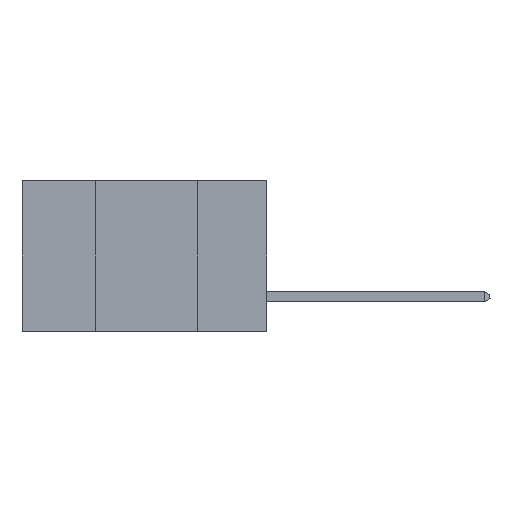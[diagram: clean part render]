
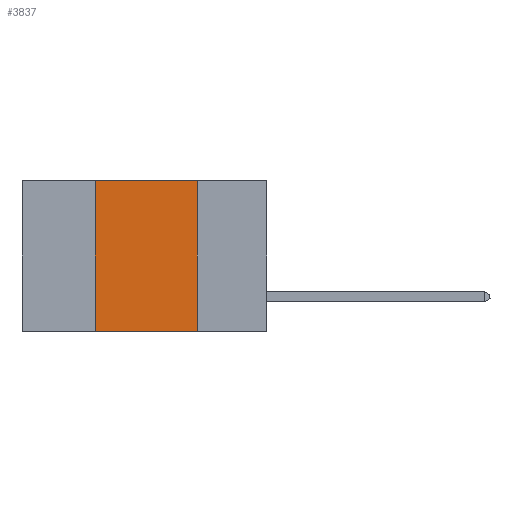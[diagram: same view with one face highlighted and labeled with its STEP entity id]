
A CAD part, left-side view. The second image highlights one B-rep face of the part: STEP entity #3837.
In plain terms, the highlighted planar face has unit normal (-1, 0, 0).
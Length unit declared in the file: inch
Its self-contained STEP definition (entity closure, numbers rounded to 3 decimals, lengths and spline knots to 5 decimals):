
#324 = CARTESIAN_POINT ( 'NONE',  ( 0., 0.42, 0. ) ) ;
#327 = CARTESIAN_POINT ( 'NONE',  ( 0., 0.42, -0.37 ) ) ;
#1622 = VECTOR ( 'NONE', #12497, 39.37008 ) ;
#2121 = CARTESIAN_POINT ( 'NONE',  ( 0., 0.17, 0. ) ) ;
#2590 = PLANE ( 'NONE',  #17501 ) ;
#3111 = ORIENTED_EDGE ( 'NONE', *, *, #18318, .F. ) ;
#3259 = CARTESIAN_POINT ( 'NONE',  ( 0., 0.42, 0. ) ) ;
#3837 = ADVANCED_FACE ( 'NONE', ( #7050 ), #2590, .F. ) ;
#4318 = VERTEX_POINT ( 'NONE', #2121 ) ;
#4724 = DIRECTION ( 'NONE',  ( 0., -1., 0. ) ) ;
#5685 = LINE ( 'NONE', #15489, #20625 ) ;
#5965 = LINE ( 'NONE', #324, #1622 ) ;
#6054 = DIRECTION ( 'NONE',  ( 0., 0., -1. ) ) ;
#6396 = LINE ( 'NONE', #6500, #17541 ) ;
#6500 = CARTESIAN_POINT ( 'NONE',  ( 0., 0.17, 0. ) ) ;
#7050 = FACE_OUTER_BOUND ( 'NONE', #10687, .T. ) ;
#7141 = VERTEX_POINT ( 'NONE', #3259 ) ;
#8416 = EDGE_CURVE ( 'NONE', #4318, #9882, #6396, .T. ) ;
#9678 = CARTESIAN_POINT ( 'NONE',  ( 0., 0.6, 0. ) ) ;
#9882 = VERTEX_POINT ( 'NONE', #21635 ) ;
#10262 = DIRECTION ( 'NONE',  ( 0., 0., -1. ) ) ;
#10321 = ORIENTED_EDGE ( 'NONE', *, *, #13271, .F. ) ;
#10687 = EDGE_LOOP ( 'NONE', ( #15034, #10321, #3111, #14745 ) ) ;
#12497 = DIRECTION ( 'NONE',  ( 0., 0., 1. ) ) ;
#13271 = EDGE_CURVE ( 'NONE', #7141, #4318, #19123, .T. ) ;
#14745 = ORIENTED_EDGE ( 'NONE', *, *, #18659, .T. ) ;
#15034 = ORIENTED_EDGE ( 'NONE', *, *, #8416, .F. ) ;
#15489 = CARTESIAN_POINT ( 'NONE',  ( 0., 0.6, -0.37 ) ) ;
#16081 = DIRECTION ( 'NONE',  ( 0., -1., 0. ) ) ;
#17501 = AXIS2_PLACEMENT_3D ( 'NONE', #9678, #18407, #6054 ) ;
#17541 = VECTOR ( 'NONE', #10262, 39.37008 ) ;
#17960 = VERTEX_POINT ( 'NONE', #327 ) ;
#17961 = CARTESIAN_POINT ( 'NONE',  ( 0., 0.6, 0. ) ) ;
#18318 = EDGE_CURVE ( 'NONE', #17960, #7141, #5965, .T. ) ;
#18407 = DIRECTION ( 'NONE',  ( 1., 0., 0. ) ) ;
#18659 = EDGE_CURVE ( 'NONE', #17960, #9882, #5685, .T. ) ;
#19123 = LINE ( 'NONE', #17961, #21308 ) ;
#20625 = VECTOR ( 'NONE', #4724, 39.37008 ) ;
#21308 = VECTOR ( 'NONE', #16081, 39.37008 ) ;
#21635 = CARTESIAN_POINT ( 'NONE',  ( 0., 0.17, -0.37 ) ) ;
